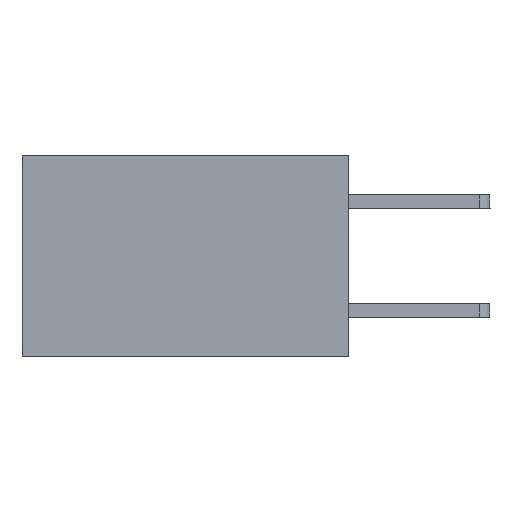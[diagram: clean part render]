
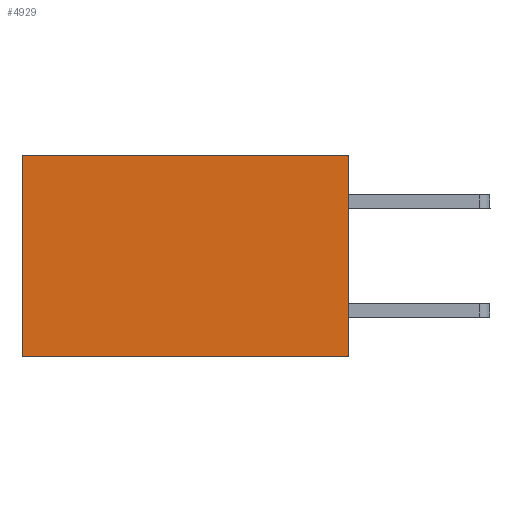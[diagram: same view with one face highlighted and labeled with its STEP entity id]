
A CAD part, left-side view. The second image highlights one B-rep face of the part: STEP entity #4929.
In plain terms, the highlighted planar face has unit normal (-1, 0, 0).
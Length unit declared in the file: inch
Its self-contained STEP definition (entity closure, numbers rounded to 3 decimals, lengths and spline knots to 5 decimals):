
#303 = FACE_OUTER_BOUND ( 'NONE', #12529, .T. ) ;
#1097 = VERTEX_POINT ( 'NONE', #10312 ) ;
#1130 = ORIENTED_EDGE ( 'NONE', *, *, #9064, .T. ) ;
#1135 = VECTOR ( 'NONE', #5723, 39.37008 ) ;
#1329 = DIRECTION ( 'NONE',  ( 0., 0., -1. ) ) ;
#1367 = EDGE_CURVE ( 'NONE', #1097, #11967, #2062, .T. ) ;
#1488 = EDGE_CURVE ( 'NONE', #4543, #11967, #3885, .T. ) ;
#1788 = LINE ( 'NONE', #8488, #1135 ) ;
#2062 = LINE ( 'NONE', #5822, #12690 ) ;
#2940 = DIRECTION ( 'NONE',  ( 0., 1., 0. ) ) ;
#3467 = CARTESIAN_POINT ( 'NONE',  ( 0.298, 0., 0. ) ) ;
#3885 = LINE ( 'NONE', #8031, #9557 ) ;
#4263 = CARTESIAN_POINT ( 'NONE',  ( 0.298, 0., 0. ) ) ;
#4543 = VERTEX_POINT ( 'NONE', #6353 ) ;
#4929 = ADVANCED_FACE ( 'NONE', ( #303 ), #10422, .F. ) ;
#5723 = DIRECTION ( 'NONE',  ( 0., 0., -1. ) ) ;
#5822 = CARTESIAN_POINT ( 'NONE',  ( 0.298, 0., -0.37 ) ) ;
#5898 = LINE ( 'NONE', #8552, #10084 ) ;
#6353 = CARTESIAN_POINT ( 'NONE',  ( 0.298, 0.6, 0. ) ) ;
#6907 = DIRECTION ( 'NONE',  ( 0., 1., 0. ) ) ;
#6980 = EDGE_CURVE ( 'NONE', #10270, #1097, #1788, .T. ) ;
#8031 = CARTESIAN_POINT ( 'NONE',  ( 0.298, 0.6, 0. ) ) ;
#8354 = AXIS2_PLACEMENT_3D ( 'NONE', #4263, #10222, #1329 ) ;
#8488 = CARTESIAN_POINT ( 'NONE',  ( 0.298, 0., 0. ) ) ;
#8552 = CARTESIAN_POINT ( 'NONE',  ( 0.298, 0., 0. ) ) ;
#9064 = EDGE_CURVE ( 'NONE', #10270, #4543, #5898, .T. ) ;
#9411 = ORIENTED_EDGE ( 'NONE', *, *, #6980, .F. ) ;
#9557 = VECTOR ( 'NONE', #11996, 39.37008 ) ;
#10084 = VECTOR ( 'NONE', #2940, 39.37008 ) ;
#10222 = DIRECTION ( 'NONE',  ( 1., 0., 0. ) ) ;
#10270 = VERTEX_POINT ( 'NONE', #3467 ) ;
#10312 = CARTESIAN_POINT ( 'NONE',  ( 0.298, 0., -0.37 ) ) ;
#10422 = PLANE ( 'NONE',  #8354 ) ;
#10780 = CARTESIAN_POINT ( 'NONE',  ( 0.298, 0.6, -0.37 ) ) ;
#11967 = VERTEX_POINT ( 'NONE', #10780 ) ;
#11996 = DIRECTION ( 'NONE',  ( 0., 0., -1. ) ) ;
#12012 = ORIENTED_EDGE ( 'NONE', *, *, #1488, .T. ) ;
#12365 = ORIENTED_EDGE ( 'NONE', *, *, #1367, .F. ) ;
#12529 = EDGE_LOOP ( 'NONE', ( #12012, #12365, #9411, #1130 ) ) ;
#12690 = VECTOR ( 'NONE', #6907, 39.37008 ) ;
